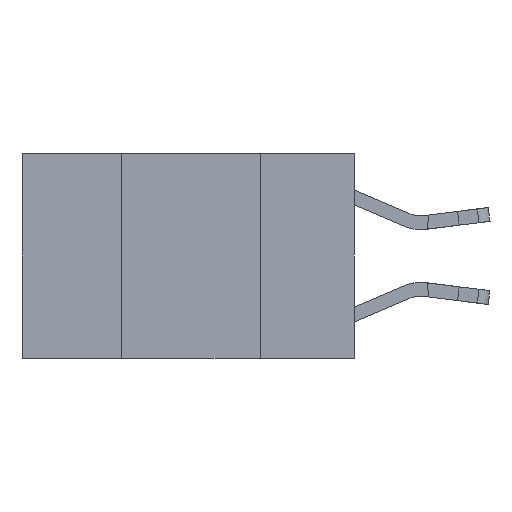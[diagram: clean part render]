
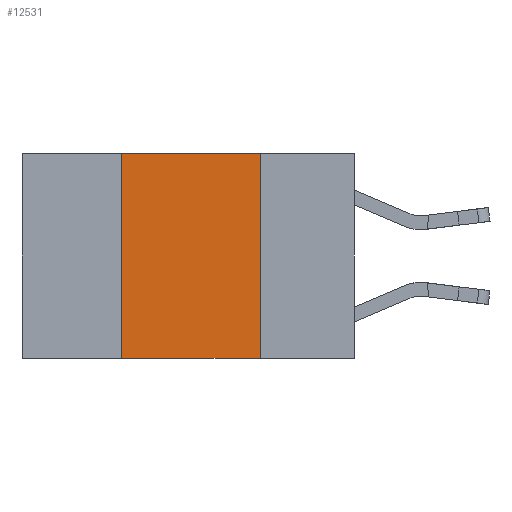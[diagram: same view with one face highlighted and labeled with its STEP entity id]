
A CAD part, left-side view. The second image highlights one B-rep face of the part: STEP entity #12531.
In plain terms, the highlighted planar face has unit normal (-1, 0, 0).
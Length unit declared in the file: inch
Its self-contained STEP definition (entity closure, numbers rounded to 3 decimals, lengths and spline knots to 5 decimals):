
#786 = EDGE_CURVE ( 'NONE', #11577, #1717, #4449, .T. ) ;
#843 = ORIENTED_EDGE ( 'NONE', *, *, #980, .F. ) ;
#980 = EDGE_CURVE ( 'NONE', #8958, #11577, #4773, .T. ) ;
#1269 = VECTOR ( 'NONE', #11452, 39.37008 ) ;
#1339 = CARTESIAN_POINT ( 'NONE',  ( 0., 0.17, -0.37 ) ) ;
#1717 = VERTEX_POINT ( 'NONE', #1339 ) ;
#2624 = ORIENTED_EDGE ( 'NONE', *, *, #786, .F. ) ;
#3121 = EDGE_CURVE ( 'NONE', #12899, #8958, #15003, .T. ) ;
#3361 = CARTESIAN_POINT ( 'NONE',  ( 0., 0.17, 0. ) ) ;
#3386 = ORIENTED_EDGE ( 'NONE', *, *, #7429, .T. ) ;
#4315 = EDGE_LOOP ( 'NONE', ( #2624, #843, #9672, #3386 ) ) ;
#4449 = LINE ( 'NONE', #3361, #11969 ) ;
#4600 = CARTESIAN_POINT ( 'NONE',  ( 0., 0.6, -0.37 ) ) ;
#4626 = DIRECTION ( 'NONE',  ( 1., 0., 0. ) ) ;
#4773 = LINE ( 'NONE', #14208, #10600 ) ;
#5442 = CARTESIAN_POINT ( 'NONE',  ( 0., 0.42, -0.37 ) ) ;
#7429 = EDGE_CURVE ( 'NONE', #12899, #1717, #9314, .T. ) ;
#7961 = CARTESIAN_POINT ( 'NONE',  ( 0., 0.42, 0. ) ) ;
#8286 = CARTESIAN_POINT ( 'NONE',  ( 0., 0.17, 0. ) ) ;
#8338 = FACE_OUTER_BOUND ( 'NONE', #4315, .T. ) ;
#8958 = VERTEX_POINT ( 'NONE', #12658 ) ;
#9314 = LINE ( 'NONE', #4600, #12365 ) ;
#9672 = ORIENTED_EDGE ( 'NONE', *, *, #3121, .F. ) ;
#10396 = DIRECTION ( 'NONE',  ( 0., 0., -1. ) ) ;
#10600 = VECTOR ( 'NONE', #11701, 39.37008 ) ;
#11452 = DIRECTION ( 'NONE',  ( 0., 0., 1. ) ) ;
#11577 = VERTEX_POINT ( 'NONE', #8286 ) ;
#11701 = DIRECTION ( 'NONE',  ( 0., -1., 0. ) ) ;
#11969 = VECTOR ( 'NONE', #14091, 39.37008 ) ;
#12365 = VECTOR ( 'NONE', #13324, 39.37008 ) ;
#12531 = ADVANCED_FACE ( 'NONE', ( #8338 ), #13043, .F. ) ;
#12658 = CARTESIAN_POINT ( 'NONE',  ( 0., 0.42, 0. ) ) ;
#12899 = VERTEX_POINT ( 'NONE', #5442 ) ;
#13043 = PLANE ( 'NONE',  #13882 ) ;
#13114 = CARTESIAN_POINT ( 'NONE',  ( 0., 0.6, 0. ) ) ;
#13324 = DIRECTION ( 'NONE',  ( 0., -1., 0. ) ) ;
#13882 = AXIS2_PLACEMENT_3D ( 'NONE', #13114, #4626, #10396 ) ;
#14091 = DIRECTION ( 'NONE',  ( 0., 0., -1. ) ) ;
#14208 = CARTESIAN_POINT ( 'NONE',  ( 0., 0.6, 0. ) ) ;
#15003 = LINE ( 'NONE', #7961, #1269 ) ;
